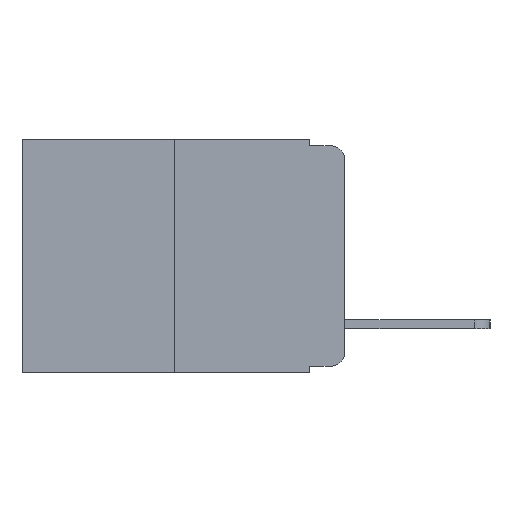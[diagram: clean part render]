
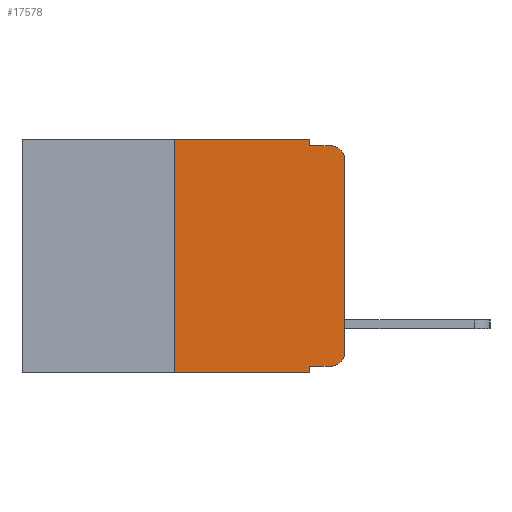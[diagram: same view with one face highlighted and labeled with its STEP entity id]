
A CAD part, left-side view. The second image highlights one B-rep face of the part: STEP entity #17578.
In plain terms, the highlighted planar face has unit normal (-1, 0, 0).
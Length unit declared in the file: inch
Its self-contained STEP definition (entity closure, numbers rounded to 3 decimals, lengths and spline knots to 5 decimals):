
#383 = VERTEX_POINT ( 'NONE', #10716 ) ;
#472 = VERTEX_POINT ( 'NONE', #19820 ) ;
#506 = EDGE_CURVE ( 'NONE', #472, #19443, #6650, .T. ) ;
#607 = CARTESIAN_POINT ( 'NONE',  ( 0., 0., -0.03 ) ) ;
#1111 = CARTESIAN_POINT ( 'NONE',  ( 0., 0.02, -0.03 ) ) ;
#1146 = CARTESIAN_POINT ( 'NONE',  ( 0., 0., 0. ) ) ;
#1319 = LINE ( 'NONE', #12499, #19103 ) ;
#1826 = LINE ( 'NONE', #10715, #10293 ) ;
#1886 = LINE ( 'NONE', #10694, #3529 ) ;
#2072 = LINE ( 'NONE', #12002, #10530 ) ;
#2156 = CARTESIAN_POINT ( 'NONE',  ( 0., 0., -0.313 ) ) ;
#2905 = DIRECTION ( 'NONE',  ( 0., 0., -1. ) ) ;
#3529 = VECTOR ( 'NONE', #20416, 39.37008 ) ;
#3723 = EDGE_CURVE ( 'NONE', #12356, #5269, #19395, .T. ) ;
#4397 = VECTOR ( 'NONE', #16858, 39.37008 ) ;
#4443 = ORIENTED_EDGE ( 'NONE', *, *, #13565, .T. ) ;
#5011 = CARTESIAN_POINT ( 'NONE',  ( 0., 0.473, 0. ) ) ;
#5269 = VERTEX_POINT ( 'NONE', #21126 ) ;
#5276 = CARTESIAN_POINT ( 'NONE',  ( 0., 0.473, 0. ) ) ;
#5412 = EDGE_CURVE ( 'NONE', #14538, #383, #1826, .T. ) ;
#5650 = CARTESIAN_POINT ( 'NONE',  ( 0., 0.051, -0.333 ) ) ;
#6061 = CARTESIAN_POINT ( 'NONE',  ( 0., 0.25, -0.343 ) ) ;
#6073 = VERTEX_POINT ( 'NONE', #6061 ) ;
#6304 = ORIENTED_EDGE ( 'NONE', *, *, #5412, .F. ) ;
#6337 = ORIENTED_EDGE ( 'NONE', *, *, #3723, .T. ) ;
#6388 = DIRECTION ( 'NONE',  ( 0., 0., 1. ) ) ;
#6562 = ORIENTED_EDGE ( 'NONE', *, *, #19529, .T. ) ;
#6650 = LINE ( 'NONE', #5276, #19273 ) ;
#6654 = DIRECTION ( 'NONE',  ( 1., 0., 0. ) ) ;
#6742 = AXIS2_PLACEMENT_3D ( 'NONE', #18610, #8755, #20089 ) ;
#7064 = EDGE_CURVE ( 'NONE', #6073, #12809, #18245, .T. ) ;
#7373 = ORIENTED_EDGE ( 'NONE', *, *, #7064, .T. ) ;
#7645 = EDGE_LOOP ( 'NONE', ( #6562, #19199, #6304, #18275, #15728, #16271, #7373, #16773, #6337, #4443 ) ) ;
#7712 = EDGE_CURVE ( 'NONE', #12356, #12809, #1319, .T. ) ;
#7797 = VERTEX_POINT ( 'NONE', #2156 ) ;
#7944 = CARTESIAN_POINT ( 'NONE',  ( 0., 0.051, 0. ) ) ;
#8421 = DIRECTION ( 'NONE',  ( 0., 0., -1. ) ) ;
#8755 = DIRECTION ( 'NONE',  ( -1., 0., 0. ) ) ;
#10293 = VECTOR ( 'NONE', #12460, 39.37008 ) ;
#10530 = VECTOR ( 'NONE', #16984, 39.37008 ) ;
#10694 = CARTESIAN_POINT ( 'NONE',  ( 0., 0.051, 0. ) ) ;
#10715 = CARTESIAN_POINT ( 'NONE',  ( 0., 0.051, -0.01 ) ) ;
#10716 = CARTESIAN_POINT ( 'NONE',  ( 0., 0.02, -0.01 ) ) ;
#10858 = CIRCLE ( 'NONE', #16356, 0.02 ) ;
#10906 = DIRECTION ( 'NONE',  ( 0., -1., 0. ) ) ;
#11895 = VERTEX_POINT ( 'NONE', #607 ) ;
#12002 = CARTESIAN_POINT ( 'NONE',  ( 0., 0.25, 0. ) ) ;
#12356 = VERTEX_POINT ( 'NONE', #5650 ) ;
#12460 = DIRECTION ( 'NONE',  ( 0., -1., 0. ) ) ;
#12499 = CARTESIAN_POINT ( 'NONE',  ( 0., 0.051, 0. ) ) ;
#12809 = VERTEX_POINT ( 'NONE', #19366 ) ;
#13013 = DIRECTION ( 'NONE',  ( -1., 0., 0. ) ) ;
#13249 = FACE_OUTER_BOUND ( 'NONE', #7645, .T. ) ;
#13565 = EDGE_CURVE ( 'NONE', #5269, #7797, #19409, .T. ) ;
#14361 = DIRECTION ( 'NONE',  ( 0., -1., 0. ) ) ;
#14367 = DIRECTION ( 'NONE',  ( 0., 0., -1. ) ) ;
#14538 = VERTEX_POINT ( 'NONE', #18878 ) ;
#15123 = CARTESIAN_POINT ( 'NONE',  ( 0., 0.051, -0.333 ) ) ;
#15149 = VECTOR ( 'NONE', #10906, 39.37008 ) ;
#15728 = ORIENTED_EDGE ( 'NONE', *, *, #506, .F. ) ;
#16271 = ORIENTED_EDGE ( 'NONE', *, *, #20739, .F. ) ;
#16356 = AXIS2_PLACEMENT_3D ( 'NONE', #1111, #13013, #2905 ) ;
#16773 = ORIENTED_EDGE ( 'NONE', *, *, #7712, .F. ) ;
#16858 = DIRECTION ( 'NONE',  ( 0., -1., 0. ) ) ;
#16984 = DIRECTION ( 'NONE',  ( 0., 0., 1. ) ) ;
#17036 = EDGE_CURVE ( 'NONE', #19443, #14538, #1886, .T. ) ;
#17454 = EDGE_CURVE ( 'NONE', #11895, #383, #10858, .T. ) ;
#17578 = ADVANCED_FACE ( 'NONE', ( #13249 ), #18336, .F. ) ;
#18245 = LINE ( 'NONE', #18709, #4397 ) ;
#18275 = ORIENTED_EDGE ( 'NONE', *, *, #17036, .F. ) ;
#18336 = PLANE ( 'NONE',  #20082 ) ;
#18610 = CARTESIAN_POINT ( 'NONE',  ( 0., 0.02, -0.313 ) ) ;
#18709 = CARTESIAN_POINT ( 'NONE',  ( 0., 0.473, -0.343 ) ) ;
#18878 = CARTESIAN_POINT ( 'NONE',  ( 0., 0.051, -0.01 ) ) ;
#19103 = VECTOR ( 'NONE', #14367, 39.37008 ) ;
#19199 = ORIENTED_EDGE ( 'NONE', *, *, #17454, .T. ) ;
#19273 = VECTOR ( 'NONE', #14361, 39.37008 ) ;
#19366 = CARTESIAN_POINT ( 'NONE',  ( 0., 0.051, -0.343 ) ) ;
#19395 = LINE ( 'NONE', #15123, #15149 ) ;
#19409 = CIRCLE ( 'NONE', #6742, 0.02 ) ;
#19443 = VERTEX_POINT ( 'NONE', #7944 ) ;
#19529 = EDGE_CURVE ( 'NONE', #7797, #11895, #21293, .T. ) ;
#19820 = CARTESIAN_POINT ( 'NONE',  ( 0., 0.25, 0. ) ) ;
#20082 = AXIS2_PLACEMENT_3D ( 'NONE', #5011, #6654, #8421 ) ;
#20089 = DIRECTION ( 'NONE',  ( 0., 0., -1. ) ) ;
#20416 = DIRECTION ( 'NONE',  ( 0., 0., -1. ) ) ;
#20739 = EDGE_CURVE ( 'NONE', #6073, #472, #2072, .T. ) ;
#20841 = VECTOR ( 'NONE', #6388, 39.37008 ) ;
#21126 = CARTESIAN_POINT ( 'NONE',  ( 0., 0.02, -0.333 ) ) ;
#21293 = LINE ( 'NONE', #1146, #20841 ) ;
